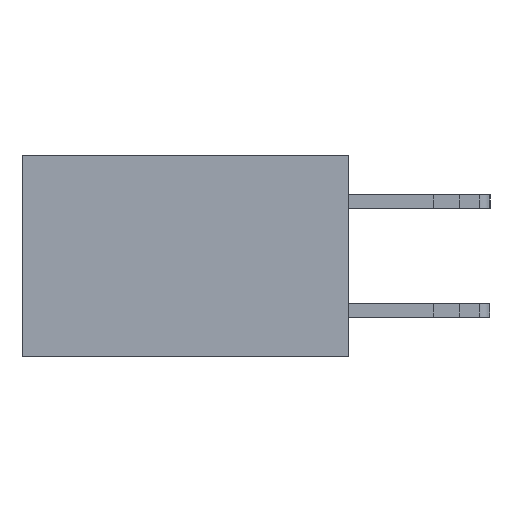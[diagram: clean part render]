
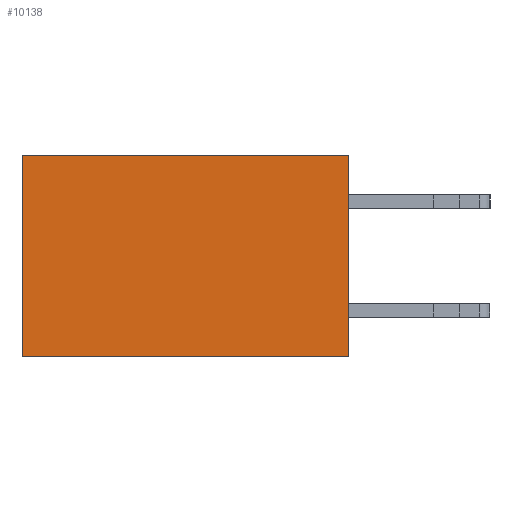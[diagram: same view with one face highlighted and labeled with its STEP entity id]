
A CAD part, left-side view. The second image highlights one B-rep face of the part: STEP entity #10138.
In plain terms, the highlighted planar face has unit normal (-1, 0, 0).
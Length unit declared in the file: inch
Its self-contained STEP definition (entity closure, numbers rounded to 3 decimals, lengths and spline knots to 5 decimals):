
#1383 = DIRECTION ( 'NONE',  ( 0., 0., -1. ) ) ;
#1955 = ORIENTED_EDGE ( 'NONE', *, *, #23904, .F. ) ;
#2072 = EDGE_CURVE ( 'NONE', #15860, #12103, #18144, .T. ) ;
#2932 = EDGE_LOOP ( 'NONE', ( #11236, #7029, #1955, #6308 ) ) ;
#4206 = VERTEX_POINT ( 'NONE', #5223 ) ;
#5223 = CARTESIAN_POINT ( 'NONE',  ( 0.298, 0., -0.37 ) ) ;
#5853 = CARTESIAN_POINT ( 'NONE',  ( 0.298, 0.6, 0. ) ) ;
#6308 = ORIENTED_EDGE ( 'NONE', *, *, #2072, .T. ) ;
#6367 = FACE_OUTER_BOUND ( 'NONE', #2932, .T. ) ;
#6702 = CARTESIAN_POINT ( 'NONE',  ( 0.298, 0.6, -0.37 ) ) ;
#7029 = ORIENTED_EDGE ( 'NONE', *, *, #17863, .F. ) ;
#7392 = VECTOR ( 'NONE', #20275, 39.37008 ) ;
#7418 = DIRECTION ( 'NONE',  ( 0., 1., 0. ) ) ;
#7986 = LINE ( 'NONE', #18372, #7392 ) ;
#8944 = PLANE ( 'NONE',  #17174 ) ;
#9010 = LINE ( 'NONE', #18608, #12855 ) ;
#10138 = ADVANCED_FACE ( 'NONE', ( #6367 ), #8944, .F. ) ;
#10844 = CARTESIAN_POINT ( 'NONE',  ( 0.298, 0., 0. ) ) ;
#11204 = CARTESIAN_POINT ( 'NONE',  ( 0.298, 0., 0. ) ) ;
#11236 = ORIENTED_EDGE ( 'NONE', *, *, #23490, .T. ) ;
#12103 = VERTEX_POINT ( 'NONE', #22780 ) ;
#12754 = DIRECTION ( 'NONE',  ( 1., 0., 0. ) ) ;
#12855 = VECTOR ( 'NONE', #7418, 39.37008 ) ;
#13022 = VECTOR ( 'NONE', #19050, 39.37008 ) ;
#15860 = VERTEX_POINT ( 'NONE', #16624 ) ;
#16624 = CARTESIAN_POINT ( 'NONE',  ( 0.298, 0., 0. ) ) ;
#16708 = DIRECTION ( 'NONE',  ( 0., 1., 0. ) ) ;
#17174 = AXIS2_PLACEMENT_3D ( 'NONE', #10844, #12754, #1383 ) ;
#17582 = VERTEX_POINT ( 'NONE', #6702 ) ;
#17863 = EDGE_CURVE ( 'NONE', #4206, #17582, #9010, .T. ) ;
#18144 = LINE ( 'NONE', #11204, #24317 ) ;
#18372 = CARTESIAN_POINT ( 'NONE',  ( 0.298, 0., 0. ) ) ;
#18608 = CARTESIAN_POINT ( 'NONE',  ( 0.298, 0., -0.37 ) ) ;
#19050 = DIRECTION ( 'NONE',  ( 0., 0., -1. ) ) ;
#20275 = DIRECTION ( 'NONE',  ( 0., 0., -1. ) ) ;
#22471 = LINE ( 'NONE', #5853, #13022 ) ;
#22780 = CARTESIAN_POINT ( 'NONE',  ( 0.298, 0.6, 0. ) ) ;
#23490 = EDGE_CURVE ( 'NONE', #12103, #17582, #22471, .T. ) ;
#23904 = EDGE_CURVE ( 'NONE', #15860, #4206, #7986, .T. ) ;
#24317 = VECTOR ( 'NONE', #16708, 39.37008 ) ;
